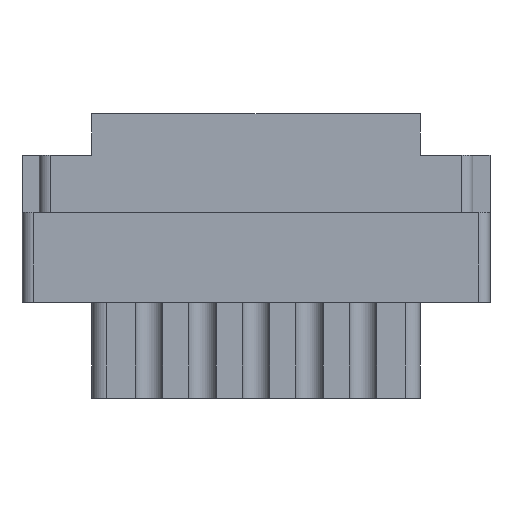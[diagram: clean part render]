
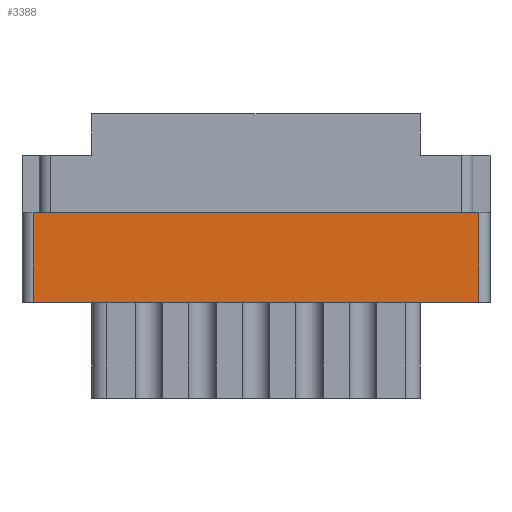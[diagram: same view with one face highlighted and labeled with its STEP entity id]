
A CAD part, front view. The second image highlights one B-rep face of the part: STEP entity #3388.
In plain terms, the highlighted planar face has unit normal (0, -1, 0).
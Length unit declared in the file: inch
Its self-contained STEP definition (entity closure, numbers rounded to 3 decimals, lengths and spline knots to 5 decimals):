
#1919 = DIRECTION ( 'NONE',  ( 0., -1., 0. ) ) ;
#2378 = CARTESIAN_POINT ( 'NONE',  ( 0.624, -0.343, -0.277 ) ) ;
#2808 = DIRECTION ( 'NONE',  ( -1., 0., 0. ) ) ;
#3388 = ADVANCED_FACE ( 'NONE', ( #11359 ), #7673, .T. ) ;
#3931 = CARTESIAN_POINT ( 'NONE',  ( -0.624, -0.343, -0.529 ) ) ;
#4350 = EDGE_CURVE ( 'NONE', #21074, #22580, #5888, .T. ) ;
#4924 = CARTESIAN_POINT ( 'NONE',  ( -0.624, -0.343, -0.798 ) ) ;
#5738 = AXIS2_PLACEMENT_3D ( 'NONE', #17356, #1919, #9854 ) ;
#5888 = LINE ( 'NONE', #20261, #17026 ) ;
#6498 = CARTESIAN_POINT ( 'NONE',  ( -0.624, -0.343, -0.277 ) ) ;
#6549 = CARTESIAN_POINT ( 'NONE',  ( 0., -0.343, -0.277 ) ) ;
#6689 = EDGE_CURVE ( 'NONE', #7885, #22580, #7275, .T. ) ;
#6924 = DIRECTION ( 'NONE',  ( 0., 0., 1. ) ) ;
#7275 = LINE ( 'NONE', #4924, #21705 ) ;
#7336 = ORIENTED_EDGE ( 'NONE', *, *, #20869, .F. ) ;
#7673 = PLANE ( 'NONE',  #5738 ) ;
#7885 = VERTEX_POINT ( 'NONE', #6498 ) ;
#8565 = DIRECTION ( 'NONE',  ( 0., 0., -1. ) ) ;
#9854 = DIRECTION ( 'NONE',  ( 0., 0., -1. ) ) ;
#10624 = VECTOR ( 'NONE', #6924, 39.37008 ) ;
#11359 = FACE_OUTER_BOUND ( 'NONE', #16409, .T. ) ;
#12229 = ORIENTED_EDGE ( 'NONE', *, *, #6689, .T. ) ;
#12682 = EDGE_CURVE ( 'NONE', #21074, #24935, #22371, .T. ) ;
#13211 = ORIENTED_EDGE ( 'NONE', *, *, #4350, .F. ) ;
#15991 = DIRECTION ( 'NONE',  ( 1., 0., 0. ) ) ;
#16409 = EDGE_LOOP ( 'NONE', ( #7336, #12229, #13211, #19264 ) ) ;
#17026 = VECTOR ( 'NONE', #2808, 39.37008 ) ;
#17356 = CARTESIAN_POINT ( 'NONE',  ( -0.656, -0.343, -0.798 ) ) ;
#18705 = CARTESIAN_POINT ( 'NONE',  ( 0.624, -0.343, -0.798 ) ) ;
#19264 = ORIENTED_EDGE ( 'NONE', *, *, #12682, .T. ) ;
#20261 = CARTESIAN_POINT ( 'NONE',  ( 0., -0.343, -0.529 ) ) ;
#20869 = EDGE_CURVE ( 'NONE', #7885, #24935, #22809, .T. ) ;
#21074 = VERTEX_POINT ( 'NONE', #24699 ) ;
#21705 = VECTOR ( 'NONE', #8565, 39.37008 ) ;
#22371 = LINE ( 'NONE', #18705, #10624 ) ;
#22580 = VERTEX_POINT ( 'NONE', #3931 ) ;
#22809 = LINE ( 'NONE', #6549, #23694 ) ;
#23694 = VECTOR ( 'NONE', #15991, 39.37008 ) ;
#24699 = CARTESIAN_POINT ( 'NONE',  ( 0.624, -0.343, -0.529 ) ) ;
#24935 = VERTEX_POINT ( 'NONE', #2378 ) ;
